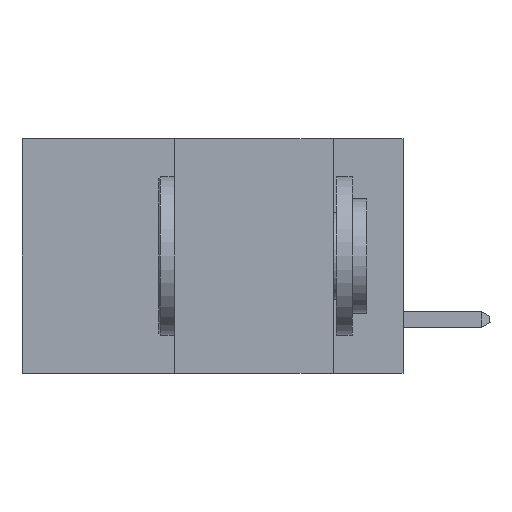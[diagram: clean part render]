
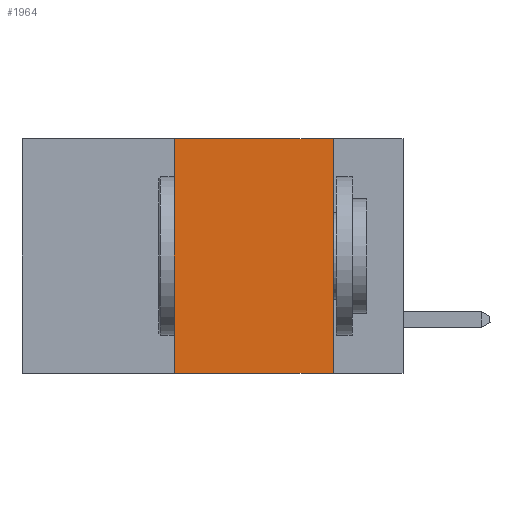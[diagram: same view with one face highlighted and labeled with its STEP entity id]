
A CAD part, left-side view. The second image highlights one B-rep face of the part: STEP entity #1964.
In plain terms, the highlighted planar face has unit normal (-1, 0, 0).
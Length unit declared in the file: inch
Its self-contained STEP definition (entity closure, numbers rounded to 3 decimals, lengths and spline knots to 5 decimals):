
#111 = VERTEX_POINT ( 'NONE', #5428 ) ;
#419 = VERTEX_POINT ( 'NONE', #9753 ) ;
#498 = EDGE_CURVE ( 'NONE', #111, #3721, #5528, .T. ) ;
#586 = FACE_OUTER_BOUND ( 'NONE', #5659, .T. ) ;
#995 = ORIENTED_EDGE ( 'NONE', *, *, #1678, .F. ) ;
#1407 = LINE ( 'NONE', #4349, #3742 ) ;
#1623 = DIRECTION ( 'NONE',  ( 0., -1., 0. ) ) ;
#1678 = EDGE_CURVE ( 'NONE', #419, #111, #8466, .T. ) ;
#1964 = ADVANCED_FACE ( 'NONE', ( #586 ), #2680, .F. ) ;
#1993 = CARTESIAN_POINT ( 'NONE',  ( 0., 0.36, 0. ) ) ;
#2680 = PLANE ( 'NONE',  #2762 ) ;
#2762 = AXIS2_PLACEMENT_3D ( 'NONE', #4435, #6767, #7537 ) ;
#3721 = VERTEX_POINT ( 'NONE', #7988 ) ;
#3742 = VECTOR ( 'NONE', #7513, 39.37008 ) ;
#4349 = CARTESIAN_POINT ( 'NONE',  ( 0., 0.6, -0.37 ) ) ;
#4435 = CARTESIAN_POINT ( 'NONE',  ( 0., 0.6, 0. ) ) ;
#4603 = CARTESIAN_POINT ( 'NONE',  ( 0., 0.6, 0. ) ) ;
#4852 = CARTESIAN_POINT ( 'NONE',  ( 0., 0.36, -0.37 ) ) ;
#5031 = ORIENTED_EDGE ( 'NONE', *, *, #8597, .T. ) ;
#5428 = CARTESIAN_POINT ( 'NONE',  ( 0., 0.11, 0. ) ) ;
#5528 = LINE ( 'NONE', #8323, #7010 ) ;
#5659 = EDGE_LOOP ( 'NONE', ( #7590, #995, #10124, #5031 ) ) ;
#6118 = VECTOR ( 'NONE', #1623, 39.37008 ) ;
#6767 = DIRECTION ( 'NONE',  ( 1., 0., 0. ) ) ;
#6944 = VERTEX_POINT ( 'NONE', #4852 ) ;
#7010 = VECTOR ( 'NONE', #8290, 39.37008 ) ;
#7418 = VECTOR ( 'NONE', #7602, 39.37008 ) ;
#7513 = DIRECTION ( 'NONE',  ( 0., -1., 0. ) ) ;
#7537 = DIRECTION ( 'NONE',  ( 0., 0., -1. ) ) ;
#7590 = ORIENTED_EDGE ( 'NONE', *, *, #498, .F. ) ;
#7602 = DIRECTION ( 'NONE',  ( 0., 0., 1. ) ) ;
#7988 = CARTESIAN_POINT ( 'NONE',  ( 0., 0.11, -0.37 ) ) ;
#8278 = LINE ( 'NONE', #1993, #7418 ) ;
#8290 = DIRECTION ( 'NONE',  ( 0., 0., -1. ) ) ;
#8323 = CARTESIAN_POINT ( 'NONE',  ( 0., 0.11, 0. ) ) ;
#8466 = LINE ( 'NONE', #4603, #6118 ) ;
#8597 = EDGE_CURVE ( 'NONE', #6944, #3721, #1407, .T. ) ;
#9434 = EDGE_CURVE ( 'NONE', #6944, #419, #8278, .T. ) ;
#9753 = CARTESIAN_POINT ( 'NONE',  ( 0., 0.36, 0. ) ) ;
#10124 = ORIENTED_EDGE ( 'NONE', *, *, #9434, .F. ) ;
